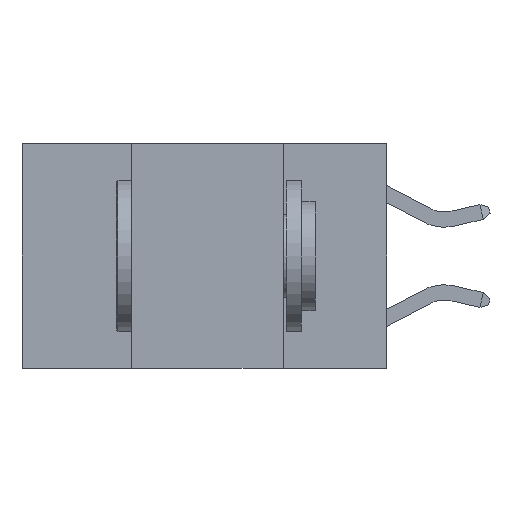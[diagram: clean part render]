
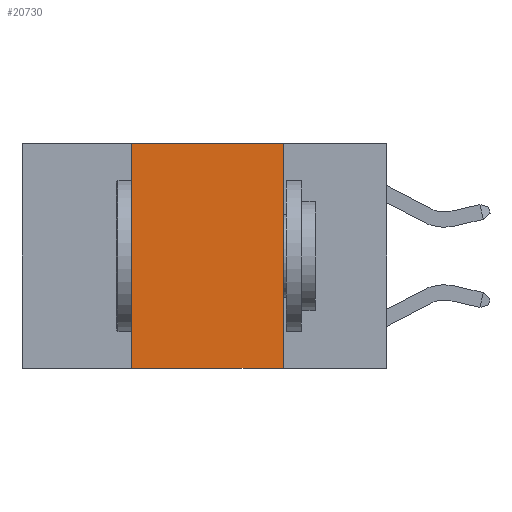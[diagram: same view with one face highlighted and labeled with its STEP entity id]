
A CAD part, left-side view. The second image highlights one B-rep face of the part: STEP entity #20730.
In plain terms, the highlighted planar face has unit normal (-1, 0, 0).
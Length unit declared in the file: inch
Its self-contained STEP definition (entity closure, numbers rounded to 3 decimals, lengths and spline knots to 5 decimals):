
#4 = VECTOR ( 'NONE', #428, 39.37008 ) ;
#428 = DIRECTION ( 'NONE',  ( 0., 0., -1. ) ) ;
#494 = CARTESIAN_POINT ( 'NONE',  ( 0., 0.42, -0.37 ) ) ;
#1258 = EDGE_CURVE ( 'NONE', #24476, #9233, #21221, .T. ) ;
#1894 = CARTESIAN_POINT ( 'NONE',  ( 0., 0.6, 0. ) ) ;
#3088 = EDGE_CURVE ( 'NONE', #24923, #20992, #5150, .T. ) ;
#3785 = ORIENTED_EDGE ( 'NONE', *, *, #23238, .F. ) ;
#3876 = DIRECTION ( 'NONE',  ( 1., 0., 0. ) ) ;
#3972 = VECTOR ( 'NONE', #17227, 39.37008 ) ;
#5150 = LINE ( 'NONE', #9833, #15583 ) ;
#5857 = LINE ( 'NONE', #13975, #4 ) ;
#6179 = VECTOR ( 'NONE', #14471, 39.37008 ) ;
#6505 = CARTESIAN_POINT ( 'NONE',  ( 0., 0.17, -0.37 ) ) ;
#7010 = EDGE_CURVE ( 'NONE', #9233, #20992, #5857, .T. ) ;
#7143 = AXIS2_PLACEMENT_3D ( 'NONE', #1894, #3876, #17589 ) ;
#7753 = ORIENTED_EDGE ( 'NONE', *, *, #1258, .F. ) ;
#8554 = CARTESIAN_POINT ( 'NONE',  ( 0., 0.6, 0. ) ) ;
#9091 = CARTESIAN_POINT ( 'NONE',  ( 0., 0.17, 0. ) ) ;
#9233 = VERTEX_POINT ( 'NONE', #9091 ) ;
#9833 = CARTESIAN_POINT ( 'NONE',  ( 0., 0.6, -0.37 ) ) ;
#10927 = FACE_OUTER_BOUND ( 'NONE', #11415, .T. ) ;
#11415 = EDGE_LOOP ( 'NONE', ( #22757, #7753, #3785, #19435 ) ) ;
#13628 = PLANE ( 'NONE',  #7143 ) ;
#13975 = CARTESIAN_POINT ( 'NONE',  ( 0., 0.17, 0. ) ) ;
#14471 = DIRECTION ( 'NONE',  ( 0., -1., 0. ) ) ;
#15583 = VECTOR ( 'NONE', #21593, 39.37008 ) ;
#17227 = DIRECTION ( 'NONE',  ( 0., 0., 1. ) ) ;
#17589 = DIRECTION ( 'NONE',  ( 0., 0., -1. ) ) ;
#19435 = ORIENTED_EDGE ( 'NONE', *, *, #3088, .T. ) ;
#20226 = LINE ( 'NONE', #24943, #3972 ) ;
#20730 = ADVANCED_FACE ( 'NONE', ( #10927 ), #13628, .F. ) ;
#20768 = CARTESIAN_POINT ( 'NONE',  ( 0., 0.42, 0. ) ) ;
#20992 = VERTEX_POINT ( 'NONE', #6505 ) ;
#21221 = LINE ( 'NONE', #8554, #6179 ) ;
#21593 = DIRECTION ( 'NONE',  ( 0., -1., 0. ) ) ;
#22757 = ORIENTED_EDGE ( 'NONE', *, *, #7010, .F. ) ;
#23238 = EDGE_CURVE ( 'NONE', #24923, #24476, #20226, .T. ) ;
#24476 = VERTEX_POINT ( 'NONE', #20768 ) ;
#24923 = VERTEX_POINT ( 'NONE', #494 ) ;
#24943 = CARTESIAN_POINT ( 'NONE',  ( 0., 0.42, 0. ) ) ;
